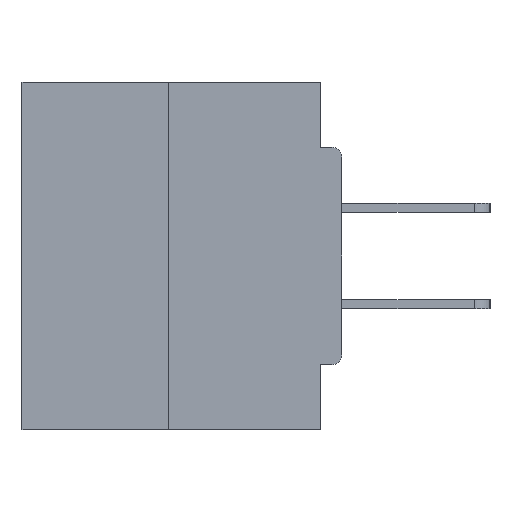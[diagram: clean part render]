
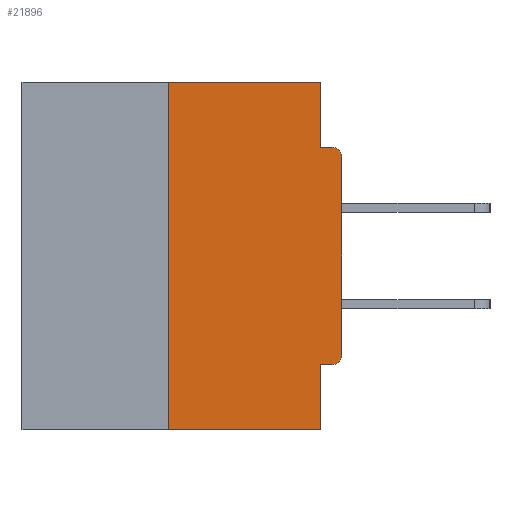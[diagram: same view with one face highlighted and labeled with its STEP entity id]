
A CAD part, left-side view. The second image highlights one B-rep face of the part: STEP entity #21896.
In plain terms, the highlighted planar face has unit normal (-1, 0, 0).
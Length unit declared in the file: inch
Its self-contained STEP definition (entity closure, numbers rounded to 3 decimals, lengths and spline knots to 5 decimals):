
#658 = VECTOR ( 'NONE', #31824, 39.37008 ) ;
#930 = EDGE_CURVE ( 'NONE', #7001, #24590, #12362, .T. ) ;
#968 = VERTEX_POINT ( 'NONE', #14906 ) ;
#1221 = FACE_OUTER_BOUND ( 'NONE', #1749, .T. ) ;
#1749 = EDGE_LOOP ( 'NONE', ( #26671, #38622, #5568, #21058, #37473, #28129, #2813, #25940, #38439, #37723 ) ) ;
#1849 = CARTESIAN_POINT ( 'NONE',  ( 0., 0.25, -0.5 ) ) ;
#2460 = VECTOR ( 'NONE', #7653, 39.37008 ) ;
#2813 = ORIENTED_EDGE ( 'NONE', *, *, #29153, .T. ) ;
#3239 = DIRECTION ( 'NONE',  ( 0., -1., 0. ) ) ;
#3557 = AXIS2_PLACEMENT_3D ( 'NONE', #4387, #28253, #7681 ) ;
#3870 = VECTOR ( 'NONE', #14914, 39.37008 ) ;
#4387 = CARTESIAN_POINT ( 'NONE',  ( 0., 0.46, 0. ) ) ;
#4938 = CARTESIAN_POINT ( 'NONE',  ( 0., 0.031, -0.5 ) ) ;
#5207 = VERTEX_POINT ( 'NONE', #1849 ) ;
#5568 = ORIENTED_EDGE ( 'NONE', *, *, #20866, .T. ) ;
#6893 = CARTESIAN_POINT ( 'NONE',  ( 0., 0.25, 0. ) ) ;
#7001 = VERTEX_POINT ( 'NONE', #9816 ) ;
#7271 = PLANE ( 'NONE',  #3557 ) ;
#7378 = LINE ( 'NONE', #32867, #38195 ) ;
#7416 = CARTESIAN_POINT ( 'NONE',  ( 0., 0.031, -0.4065 ) ) ;
#7496 = VERTEX_POINT ( 'NONE', #32955 ) ;
#7519 = CARTESIAN_POINT ( 'NONE',  ( 0., 0., 0. ) ) ;
#7653 = DIRECTION ( 'NONE',  ( 0., 0., 1. ) ) ;
#7681 = DIRECTION ( 'NONE',  ( 0., 0., -1. ) ) ;
#8680 = EDGE_CURVE ( 'NONE', #22621, #24590, #12582, .T. ) ;
#8772 = CARTESIAN_POINT ( 'NONE',  ( 0., 0.031, 0. ) ) ;
#8932 = CARTESIAN_POINT ( 'NONE',  ( 0., 0.015, -0.3915 ) ) ;
#9157 = CARTESIAN_POINT ( 'NONE',  ( 0., 0., -0.4065 ) ) ;
#9816 = CARTESIAN_POINT ( 'NONE',  ( 0., 0.031, -0.0935 ) ) ;
#10402 = LINE ( 'NONE', #7519, #2460 ) ;
#11396 = CARTESIAN_POINT ( 'NONE',  ( 0., 0.25, 0. ) ) ;
#11908 = DIRECTION ( 'NONE',  ( -1., 0., 0. ) ) ;
#12362 = LINE ( 'NONE', #32627, #23523 ) ;
#12582 = CIRCLE ( 'NONE', #17549, 0.015 ) ;
#13872 = VERTEX_POINT ( 'NONE', #6893 ) ;
#14254 = CARTESIAN_POINT ( 'NONE',  ( 0., 0.015, -0.1085 ) ) ;
#14906 = CARTESIAN_POINT ( 'NONE',  ( 0., 0.031, 0. ) ) ;
#14914 = DIRECTION ( 'NONE',  ( 0., 1., 0. ) ) ;
#15872 = LINE ( 'NONE', #20229, #27059 ) ;
#16863 = VERTEX_POINT ( 'NONE', #37848 ) ;
#17111 = DIRECTION ( 'NONE',  ( 0., 0., -1. ) ) ;
#17237 = DIRECTION ( 'NONE',  ( 0., 0., -1. ) ) ;
#17549 = AXIS2_PLACEMENT_3D ( 'NONE', #14254, #35087, #17237 ) ;
#17976 = EDGE_CURVE ( 'NONE', #7496, #20392, #19763, .T. ) ;
#18702 = EDGE_CURVE ( 'NONE', #968, #7001, #29495, .T. ) ;
#19561 = CIRCLE ( 'NONE', #30635, 0.015 ) ;
#19763 = LINE ( 'NONE', #9157, #3870 ) ;
#19829 = EDGE_CURVE ( 'NONE', #13872, #968, #15872, .T. ) ;
#20229 = CARTESIAN_POINT ( 'NONE',  ( 0., 0.46, 0. ) ) ;
#20392 = VERTEX_POINT ( 'NONE', #7416 ) ;
#20866 = EDGE_CURVE ( 'NONE', #5207, #28850, #7378, .T. ) ;
#21058 = ORIENTED_EDGE ( 'NONE', *, *, #37961, .F. ) ;
#21583 = CARTESIAN_POINT ( 'NONE',  ( 0., 0.031, -0.5 ) ) ;
#21896 = ADVANCED_FACE ( 'NONE', ( #1221 ), #7271, .F. ) ;
#22621 = VERTEX_POINT ( 'NONE', #37634 ) ;
#23523 = VECTOR ( 'NONE', #33128, 39.37008 ) ;
#24590 = VERTEX_POINT ( 'NONE', #33821 ) ;
#25002 = EDGE_CURVE ( 'NONE', #7496, #16863, #19561, .T. ) ;
#25539 = EDGE_CURVE ( 'NONE', #5207, #13872, #30212, .T. ) ;
#25940 = ORIENTED_EDGE ( 'NONE', *, *, #8680, .T. ) ;
#26671 = ORIENTED_EDGE ( 'NONE', *, *, #19829, .F. ) ;
#27059 = VECTOR ( 'NONE', #34835, 39.37008 ) ;
#28129 = ORIENTED_EDGE ( 'NONE', *, *, #25002, .T. ) ;
#28253 = DIRECTION ( 'NONE',  ( 1., 0., 0. ) ) ;
#28850 = VERTEX_POINT ( 'NONE', #21583 ) ;
#29153 = EDGE_CURVE ( 'NONE', #16863, #22621, #10402, .T. ) ;
#29495 = LINE ( 'NONE', #8772, #37905 ) ;
#30212 = LINE ( 'NONE', #11396, #33953 ) ;
#30635 = AXIS2_PLACEMENT_3D ( 'NONE', #8932, #11908, #32785 ) ;
#31824 = DIRECTION ( 'NONE',  ( 0., 0., -1. ) ) ;
#31919 = LINE ( 'NONE', #4938, #658 ) ;
#32627 = CARTESIAN_POINT ( 'NONE',  ( 0., 0., -0.0935 ) ) ;
#32785 = DIRECTION ( 'NONE',  ( 0., 0., -1. ) ) ;
#32867 = CARTESIAN_POINT ( 'NONE',  ( 0., 0.46, -0.5 ) ) ;
#32955 = CARTESIAN_POINT ( 'NONE',  ( 0., 0.015, -0.4065 ) ) ;
#33128 = DIRECTION ( 'NONE',  ( 0., -1., 0. ) ) ;
#33821 = CARTESIAN_POINT ( 'NONE',  ( 0., 0.015, -0.0935 ) ) ;
#33953 = VECTOR ( 'NONE', #38137, 39.37008 ) ;
#34835 = DIRECTION ( 'NONE',  ( 0., -1., 0. ) ) ;
#35087 = DIRECTION ( 'NONE',  ( -1., 0., 0. ) ) ;
#37473 = ORIENTED_EDGE ( 'NONE', *, *, #17976, .F. ) ;
#37634 = CARTESIAN_POINT ( 'NONE',  ( 0., 0., -0.1085 ) ) ;
#37723 = ORIENTED_EDGE ( 'NONE', *, *, #18702, .F. ) ;
#37848 = CARTESIAN_POINT ( 'NONE',  ( 0., 0., -0.3915 ) ) ;
#37905 = VECTOR ( 'NONE', #17111, 39.37008 ) ;
#37961 = EDGE_CURVE ( 'NONE', #20392, #28850, #31919, .T. ) ;
#38137 = DIRECTION ( 'NONE',  ( 0., 0., 1. ) ) ;
#38195 = VECTOR ( 'NONE', #3239, 39.37008 ) ;
#38439 = ORIENTED_EDGE ( 'NONE', *, *, #930, .F. ) ;
#38622 = ORIENTED_EDGE ( 'NONE', *, *, #25539, .F. ) ;
